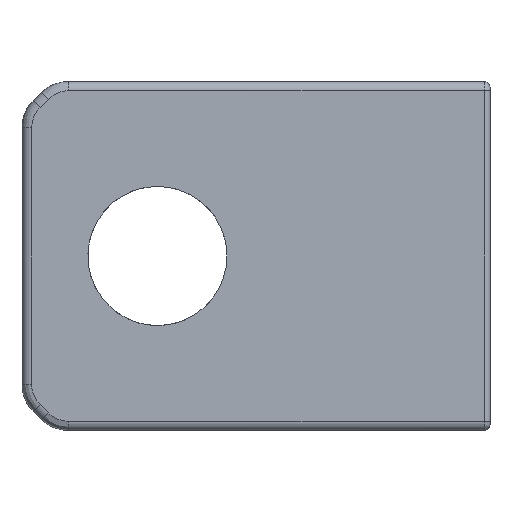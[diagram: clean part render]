
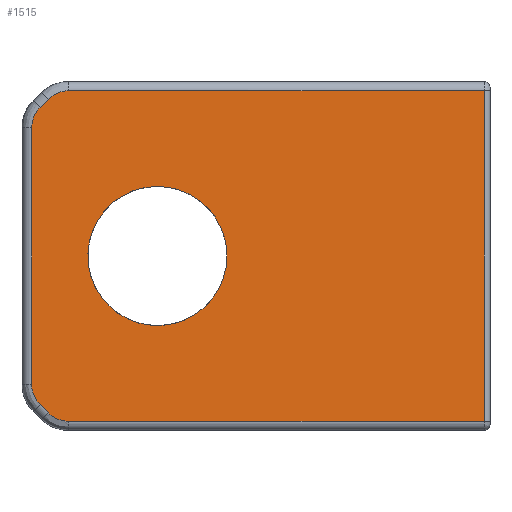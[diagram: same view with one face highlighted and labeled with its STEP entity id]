
A CAD part, front view. The second image highlights one B-rep face of the part: STEP entity #1515.
In plain terms, the highlighted planar face has unit normal (0.07, -0.998, 0).
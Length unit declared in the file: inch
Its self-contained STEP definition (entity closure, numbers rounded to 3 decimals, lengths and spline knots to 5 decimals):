
#21=FACE_BOUND('',#517,.T.);
#41=PLANE('',#1685);
#108=ELLIPSE('',#1686,0.09523,0.095);
#109=ELLIPSE('',#1687,0.09523,0.095);
#110=ELLIPSE('',#1688,0.09523,0.095);
#111=ELLIPSE('',#1689,0.09523,0.095);
#112=ELLIPSE('',#1690,0.23056,0.23);
#129=LINE('',#2336,#232);
#168=LINE('',#2806,#271);
#169=LINE('',#2810,#272);
#170=LINE('',#2814,#273);
#171=LINE('',#2818,#274);
#172=LINE('',#2822,#275);
#232=VECTOR('',#1828,0.3937);
#271=VECTOR('',#2017,0.3937);
#272=VECTOR('',#2022,0.3937);
#273=VECTOR('',#2025,0.3937);
#274=VECTOR('',#2028,0.3937);
#275=VECTOR('',#2031,0.3937);
#419=FACE_OUTER_BOUND('',#516,.T.);
#516=EDGE_LOOP('',(#1180,#1181,#1182,#1183,#1184,#1185,#1186,#1187,#1188,
#1189));
#517=EDGE_LOOP('',(#1190));
#654=VERTEX_POINT('',#2326);
#656=VERTEX_POINT('',#2332);
#714=VERTEX_POINT('',#2805);
#715=VERTEX_POINT('',#2809);
#716=VERTEX_POINT('',#2811);
#717=VERTEX_POINT('',#2813);
#718=VERTEX_POINT('',#2815);
#719=VERTEX_POINT('',#2817);
#720=VERTEX_POINT('',#2819);
#721=VERTEX_POINT('',#2821);
#722=VERTEX_POINT('',#2824);
#798=EDGE_CURVE('',#654,#656,#129,.T.);
#892=EDGE_CURVE('',#656,#714,#168,.T.);
#894=EDGE_CURVE('',#715,#654,#169,.T.);
#895=EDGE_CURVE('',#716,#715,#108,.T.);
#896=EDGE_CURVE('',#717,#716,#170,.T.);
#897=EDGE_CURVE('',#718,#717,#109,.T.);
#898=EDGE_CURVE('',#719,#718,#171,.T.);
#899=EDGE_CURVE('',#720,#719,#110,.T.);
#900=EDGE_CURVE('',#721,#720,#172,.T.);
#901=EDGE_CURVE('',#714,#721,#111,.T.);
#902=EDGE_CURVE('',#722,#722,#112,.T.);
#1180=ORIENTED_EDGE('',*,*,#798,.F.);
#1181=ORIENTED_EDGE('',*,*,#894,.F.);
#1182=ORIENTED_EDGE('',*,*,#895,.F.);
#1183=ORIENTED_EDGE('',*,*,#896,.F.);
#1184=ORIENTED_EDGE('',*,*,#897,.F.);
#1185=ORIENTED_EDGE('',*,*,#898,.F.);
#1186=ORIENTED_EDGE('',*,*,#899,.F.);
#1187=ORIENTED_EDGE('',*,*,#900,.F.);
#1188=ORIENTED_EDGE('',*,*,#901,.F.);
#1189=ORIENTED_EDGE('',*,*,#892,.F.);
#1190=ORIENTED_EDGE('',*,*,#902,.T.);
#1515=ADVANCED_FACE('',(#419,#21),#41,.F.);
#1685=AXIS2_PLACEMENT_3D('',#2808,#2020,#2021);
#1686=AXIS2_PLACEMENT_3D('',#2812,#2023,#2024);
#1687=AXIS2_PLACEMENT_3D('',#2816,#2026,#2027);
#1688=AXIS2_PLACEMENT_3D('',#2820,#2029,#2030);
#1689=AXIS2_PLACEMENT_3D('',#2823,#2032,#2033);
#1690=AXIS2_PLACEMENT_3D('',#2825,#2034,#2035);
#1828=DIRECTION('',(0.,0.,-1.));
#2017=DIRECTION('',(-0.998,-0.07,0.));
#2020=DIRECTION('center_axis',(-0.07,0.998,0.));
#2021=DIRECTION('ref_axis',(0.,0.,1.));
#2022=DIRECTION('',(0.998,0.07,0.));
#2023=DIRECTION('center_axis',(-0.07,0.998,0.));
#2024=DIRECTION('ref_axis',(-0.998,-0.07,0.));
#2025=DIRECTION('',(0.706,0.05,0.706));
#2026=DIRECTION('center_axis',(-0.07,0.998,0.));
#2027=DIRECTION('ref_axis',(-0.998,-0.07,0.));
#2028=DIRECTION('',(0.,0.,1.));
#2029=DIRECTION('center_axis',(-0.07,0.998,0.));
#2030=DIRECTION('ref_axis',(-0.998,-0.07,0.));
#2031=DIRECTION('',(-0.706,-0.05,0.706));
#2032=DIRECTION('center_axis',(-0.07,0.998,0.));
#2033=DIRECTION('ref_axis',(-0.998,-0.07,0.));
#2034=DIRECTION('center_axis',(-0.07,0.998,0.));
#2035=DIRECTION('ref_axis',(-0.998,-0.07,0.));
#2326=CARTESIAN_POINT('',(1.5294,-0.0006,-0.02));
#2332=CARTESIAN_POINT('',(1.5294,-0.0006,-1.113));
#2336=CARTESIAN_POINT('',(1.5294,-0.0006,-0.28325));
#2805=CARTESIAN_POINT('',(0.15387,-0.09705,-1.113));
#2806=CARTESIAN_POINT('',(1.16104,-0.02643,-1.113));
#2808=CARTESIAN_POINT('Origin',(0.77412,-0.05356,-0.5665));
#2809=CARTESIAN_POINT('',(0.15387,-0.09705,-0.02));
#2810=CARTESIAN_POINT('',(0.39082,-0.08043,-0.02));
#2811=CARTESIAN_POINT('',(0.0867,-0.10176,-0.04782));
#2812=CARTESIAN_POINT('Origin',(0.15387,-0.09705,-0.115));
#2813=CARTESIAN_POINT('',(0.05992,-0.10364,-0.0746));
#2814=CARTESIAN_POINT('',(0.1242,-0.09913,-0.01032));
#2815=CARTESIAN_POINT('',(0.0321,-0.10559,-0.14178));
#2816=CARTESIAN_POINT('Origin',(0.1271,-0.09893,-0.14178));
#2817=CARTESIAN_POINT('',(0.0321,-0.10559,-0.99122));
#2818=CARTESIAN_POINT('',(0.0321,-0.10559,-0.84975));
#2819=CARTESIAN_POINT('',(0.05992,-0.10364,-1.0584));
#2820=CARTESIAN_POINT('Origin',(0.1271,-0.09893,-0.99122));
#2821=CARTESIAN_POINT('',(0.0867,-0.10176,-1.08518));
#2822=CARTESIAN_POINT('',(0.1242,-0.09913,-1.12268));
#2823=CARTESIAN_POINT('Origin',(0.15387,-0.09705,-1.018));
#2824=CARTESIAN_POINT('',(0.678,-0.0603,-0.5665));
#2825=CARTESIAN_POINT('Origin',(0.448,-0.07643,-0.5665));
